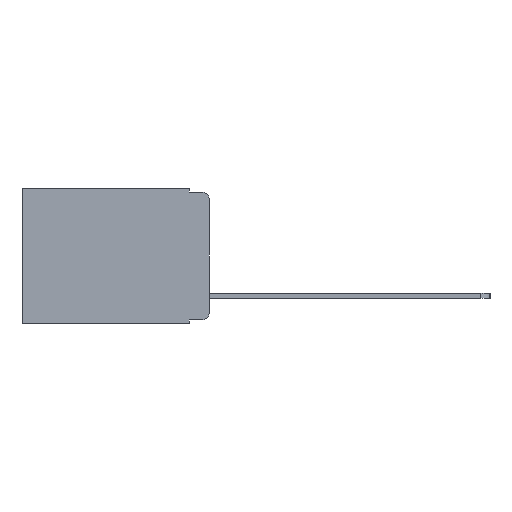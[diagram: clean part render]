
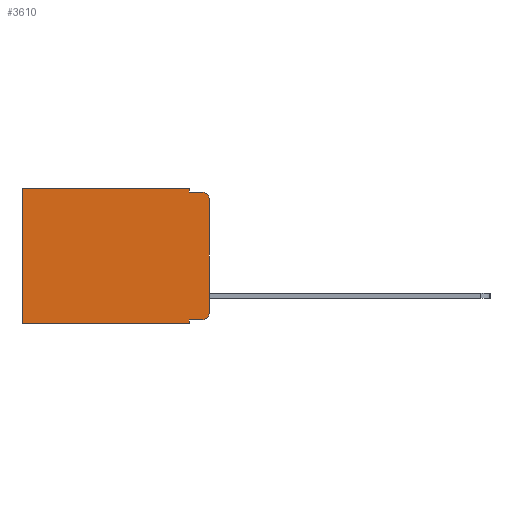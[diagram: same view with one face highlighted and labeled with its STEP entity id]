
A CAD part, left-side view. The second image highlights one B-rep face of the part: STEP entity #3610.
In plain terms, the highlighted planar face has unit normal (-1, 0, 0).
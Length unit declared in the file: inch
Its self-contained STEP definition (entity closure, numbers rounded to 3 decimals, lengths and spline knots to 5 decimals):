
#303 = AXIS2_PLACEMENT_3D ( 'NONE', #8512, #7777, #939 ) ;
#339 = VERTEX_POINT ( 'NONE', #5587 ) ;
#350 = ORIENTED_EDGE ( 'NONE', *, *, #1153, .F. ) ;
#377 = VECTOR ( 'NONE', #1152, 39.37008 ) ;
#389 = PLANE ( 'NONE',  #3280 ) ;
#390 = ORIENTED_EDGE ( 'NONE', *, *, #3501, .T. ) ;
#407 = DIRECTION ( 'NONE',  ( 0., 0., -1. ) ) ;
#669 = LINE ( 'NONE', #8704, #9484 ) ;
#675 = ORIENTED_EDGE ( 'NONE', *, *, #5814, .F. ) ;
#939 = DIRECTION ( 'NONE',  ( 0., 0., -1. ) ) ;
#953 = LINE ( 'NONE', #2204, #5329 ) ;
#1152 = DIRECTION ( 'NONE',  ( 0., 1., 0. ) ) ;
#1153 = EDGE_CURVE ( 'NONE', #7861, #4061, #3529, .T. ) ;
#1189 = VECTOR ( 'NONE', #1762, 39.37008 ) ;
#1762 = DIRECTION ( 'NONE',  ( 0., -1., 0. ) ) ;
#1803 = DIRECTION ( 'NONE',  ( -1., 0., 0. ) ) ;
#2074 = LINE ( 'NONE', #8017, #4424 ) ;
#2204 = CARTESIAN_POINT ( 'NONE',  ( 0.298, 0.051, 0. ) ) ;
#2480 = CARTESIAN_POINT ( 'NONE',  ( 0.298, 0., -0.313 ) ) ;
#2713 = DIRECTION ( 'NONE',  ( 1., 0., 0. ) ) ;
#2728 = DIRECTION ( 'NONE',  ( 0., 0., -1. ) ) ;
#2731 = LINE ( 'NONE', #5304, #6742 ) ;
#2781 = CARTESIAN_POINT ( 'NONE',  ( 0.298, 0.051, -0.01 ) ) ;
#2803 = VERTEX_POINT ( 'NONE', #4026 ) ;
#3014 = CARTESIAN_POINT ( 'NONE',  ( 0.298, 0.02, -0.333 ) ) ;
#3114 = ORIENTED_EDGE ( 'NONE', *, *, #9462, .F. ) ;
#3261 = CARTESIAN_POINT ( 'NONE',  ( 0.298, 0., 0. ) ) ;
#3280 = AXIS2_PLACEMENT_3D ( 'NONE', #4679, #2713, #2728 ) ;
#3501 = EDGE_CURVE ( 'NONE', #339, #4061, #6405, .T. ) ;
#3529 = LINE ( 'NONE', #2781, #1189 ) ;
#3569 = DIRECTION ( 'NONE',  ( 0., 0., -1. ) ) ;
#3610 = ADVANCED_FACE ( 'NONE', ( #7811 ), #389, .F. ) ;
#3832 = DIRECTION ( 'NONE',  ( 0., 0., -1. ) ) ;
#4026 = CARTESIAN_POINT ( 'NONE',  ( 0.298, 0.051, 0. ) ) ;
#4061 = VERTEX_POINT ( 'NONE', #8741 ) ;
#4102 = EDGE_LOOP ( 'NONE', ( #675, #390, #350, #9449, #6470, #9825, #10328, #3114, #9038, #7676 ) ) ;
#4424 = VECTOR ( 'NONE', #3832, 39.37008 ) ;
#4448 = CARTESIAN_POINT ( 'NONE',  ( 0.298, 0., -0.343 ) ) ;
#4483 = CARTESIAN_POINT ( 'NONE',  ( 0.298, 0.051, -0.01 ) ) ;
#4679 = CARTESIAN_POINT ( 'NONE',  ( 0.298, 0., 0. ) ) ;
#4845 = LINE ( 'NONE', #4448, #8989 ) ;
#4972 = DIRECTION ( 'NONE',  ( 0., 0., -1. ) ) ;
#5280 = DIRECTION ( 'NONE',  ( 0., 1., 0. ) ) ;
#5304 = CARTESIAN_POINT ( 'NONE',  ( 0.298, 0.051, 0. ) ) ;
#5329 = VECTOR ( 'NONE', #407, 39.37008 ) ;
#5406 = DIRECTION ( 'NONE',  ( 0., -1., 0. ) ) ;
#5587 = CARTESIAN_POINT ( 'NONE',  ( 0.298, 0., -0.03 ) ) ;
#5664 = CARTESIAN_POINT ( 'NONE',  ( 0.298, 0.473, -0.343 ) ) ;
#5814 = EDGE_CURVE ( 'NONE', #339, #9001, #8177, .T. ) ;
#5926 = VERTEX_POINT ( 'NONE', #6819 ) ;
#5994 = VECTOR ( 'NONE', #4972, 39.37008 ) ;
#6127 = EDGE_CURVE ( 'NONE', #6757, #6814, #669, .T. ) ;
#6405 = CIRCLE ( 'NONE', #303, 0.02 ) ;
#6470 = ORIENTED_EDGE ( 'NONE', *, *, #9923, .T. ) ;
#6742 = VECTOR ( 'NONE', #3569, 39.37008 ) ;
#6757 = VERTEX_POINT ( 'NONE', #10474 ) ;
#6814 = VERTEX_POINT ( 'NONE', #3014 ) ;
#6819 = CARTESIAN_POINT ( 'NONE',  ( 0.298, 0.051, -0.343 ) ) ;
#6928 = CARTESIAN_POINT ( 'NONE',  ( 0.298, 0.02, -0.313 ) ) ;
#7012 = LINE ( 'NONE', #7157, #377 ) ;
#7157 = CARTESIAN_POINT ( 'NONE',  ( 0.298, 0., 0. ) ) ;
#7676 = ORIENTED_EDGE ( 'NONE', *, *, #9104, .T. ) ;
#7748 = DIRECTION ( 'NONE',  ( 0., 0., -1. ) ) ;
#7777 = DIRECTION ( 'NONE',  ( -1., 0., 0. ) ) ;
#7811 = FACE_OUTER_BOUND ( 'NONE', #4102, .T. ) ;
#7830 = EDGE_CURVE ( 'NONE', #5926, #8815, #4845, .T. ) ;
#7861 = VERTEX_POINT ( 'NONE', #4483 ) ;
#8017 = CARTESIAN_POINT ( 'NONE',  ( 0.298, 0.473, 0. ) ) ;
#8177 = LINE ( 'NONE', #3261, #5994 ) ;
#8512 = CARTESIAN_POINT ( 'NONE',  ( 0.298, 0.02, -0.03 ) ) ;
#8704 = CARTESIAN_POINT ( 'NONE',  ( 0.298, 0.051, -0.333 ) ) ;
#8741 = CARTESIAN_POINT ( 'NONE',  ( 0.298, 0.02, -0.01 ) ) ;
#8775 = VERTEX_POINT ( 'NONE', #9745 ) ;
#8815 = VERTEX_POINT ( 'NONE', #5664 ) ;
#8962 = CIRCLE ( 'NONE', #10920, 0.02 ) ;
#8989 = VECTOR ( 'NONE', #5280, 39.37008 ) ;
#9001 = VERTEX_POINT ( 'NONE', #2480 ) ;
#9038 = ORIENTED_EDGE ( 'NONE', *, *, #6127, .T. ) ;
#9104 = EDGE_CURVE ( 'NONE', #6814, #9001, #8962, .T. ) ;
#9357 = EDGE_CURVE ( 'NONE', #8775, #8815, #2074, .T. ) ;
#9449 = ORIENTED_EDGE ( 'NONE', *, *, #10427, .F. ) ;
#9462 = EDGE_CURVE ( 'NONE', #6757, #5926, #953, .T. ) ;
#9484 = VECTOR ( 'NONE', #5406, 39.37008 ) ;
#9745 = CARTESIAN_POINT ( 'NONE',  ( 0.298, 0.473, 0. ) ) ;
#9825 = ORIENTED_EDGE ( 'NONE', *, *, #9357, .T. ) ;
#9923 = EDGE_CURVE ( 'NONE', #2803, #8775, #7012, .T. ) ;
#10328 = ORIENTED_EDGE ( 'NONE', *, *, #7830, .F. ) ;
#10427 = EDGE_CURVE ( 'NONE', #2803, #7861, #2731, .T. ) ;
#10474 = CARTESIAN_POINT ( 'NONE',  ( 0.298, 0.051, -0.333 ) ) ;
#10920 = AXIS2_PLACEMENT_3D ( 'NONE', #6928, #1803, #7748 ) ;
